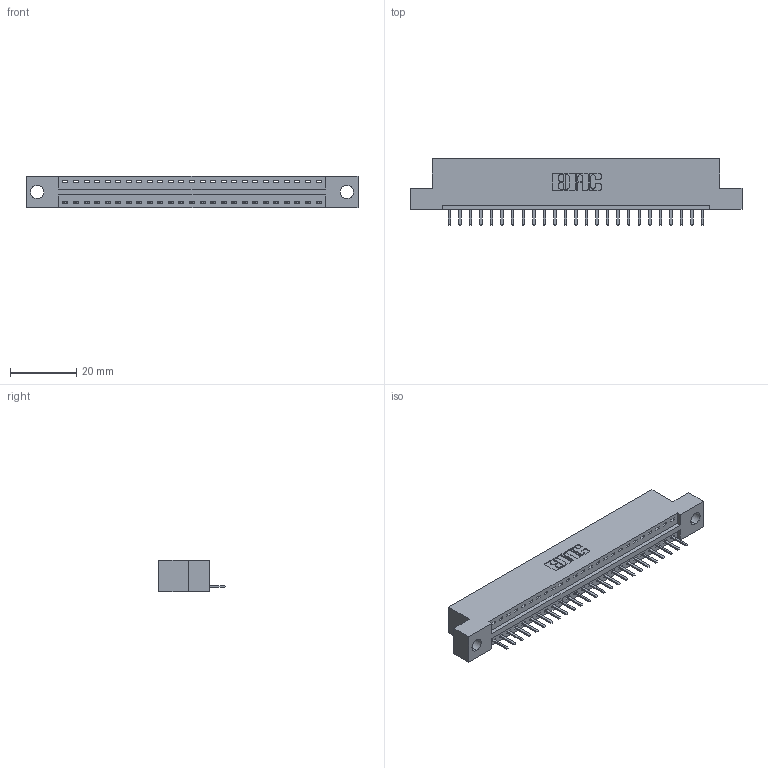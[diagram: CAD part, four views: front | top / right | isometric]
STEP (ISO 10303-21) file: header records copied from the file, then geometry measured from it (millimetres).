
FILE_DESCRIPTION (( 'STEP AP203' ), '1' );
FILE_NAME ('396-025-520-104.STEP', '2018-09-01T15:51:05', ( '' ), ( '' ), 'SwSTEP 2.0', 'SolidWorks 2016', '' );
FILE_SCHEMA (( 'CONFIG_CONTROL_DESIGN' ));
Length unit declared in the file: inch
Products named in the file (3): 396-025-520-104; 346 Part_Flush Mounting Lugs - 0.156 Dia-TH; 345-292-001_345-293-120
Assembly tree (26 placements, depth 2):
  396-025-520-104
    346 Part_Flush Mounting Lugs - 0.156 Dia-TH
    345-292-001_345-293-120  x25
Bounding box: 99.95 x 20.02 x 9.4 mm (x, y, z)
Volume: 9290.4 mm3; surface area: 10993.3 mm2
Topology: 26 solids, 26 shells, 1672 faces, 4929 edges, 3218 vertices
Faces by surface type: plane 1126, cylinder 546
Entity records: 17921 total; most frequent: CARTESIAN_POINT 3095, ORIENTED_EDGE 3042, DIRECTION 2739, EDGE_CURVE 1521, VECTOR 1285, LINE 1285, VERTEX_POINT 1010, AXIS2_PLACEMENT_3D 727
